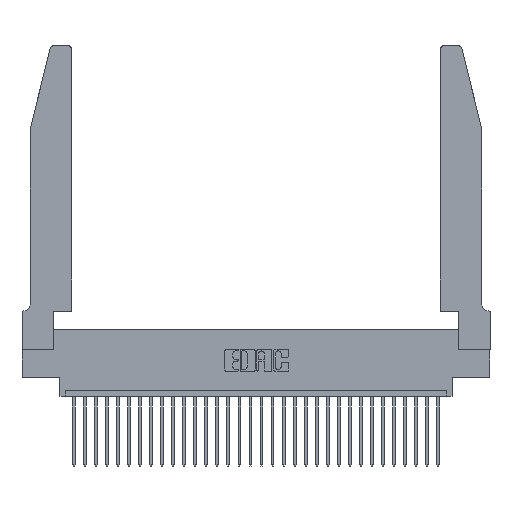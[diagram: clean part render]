
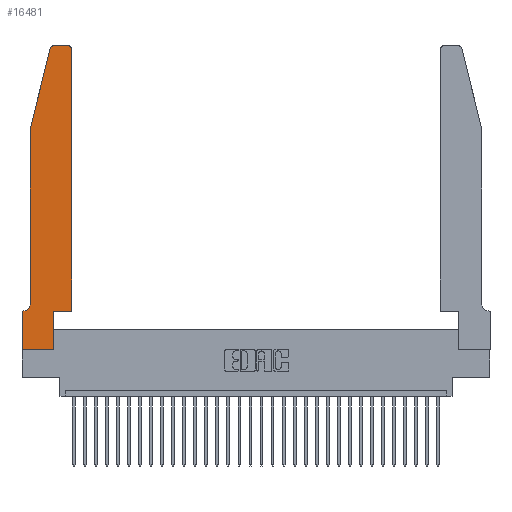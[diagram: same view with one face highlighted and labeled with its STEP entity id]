
A CAD part, top view. The second image highlights one B-rep face of the part: STEP entity #16481.
In plain terms, the highlighted planar face has unit normal (0, 0, 1).
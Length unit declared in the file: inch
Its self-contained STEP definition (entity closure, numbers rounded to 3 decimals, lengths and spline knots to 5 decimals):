
#153 = CARTESIAN_POINT ( 'NONE',  ( 0.0755, 2., 0.37 ) ) ;
#280 = CARTESIAN_POINT ( 'NONE',  ( 0.0055, 0.35, 0.37 ) ) ;
#461 = CIRCLE ( 'NONE', #27323, 0.07 ) ;
#465 = EDGE_CURVE ( 'NONE', #18346, #7004, #461, .T. ) ;
#508 = CARTESIAN_POINT ( 'NONE',  ( 0.284, 2.75, 0.37 ) ) ;
#519 = CARTESIAN_POINT ( 'NONE',  ( 0.2865, 0.35, 0.37 ) ) ;
#1228 = CARTESIAN_POINT ( 'NONE',  ( 0., 0., 0.37 ) ) ;
#1520 = VERTEX_POINT ( 'NONE', #13369 ) ;
#1771 = VECTOR ( 'NONE', #6587, 39.37008 ) ;
#2228 = CARTESIAN_POINT ( 'NONE',  ( 0.2865, 0., 0.37 ) ) ;
#2359 = DIRECTION ( 'NONE',  ( 0., 1., 0. ) ) ;
#2388 = EDGE_CURVE ( 'NONE', #21595, #28389, #28899, .T. ) ;
#2615 = CARTESIAN_POINT ( 'NONE',  ( 0.4205, 2.75, 0.37 ) ) ;
#2715 = DIRECTION ( 'NONE',  ( 1., 0., 0. ) ) ;
#3017 = DIRECTION ( 'NONE',  ( 0., 0., 1. ) ) ;
#3355 = CARTESIAN_POINT ( 'NONE',  ( 0., 0., 0.37 ) ) ;
#3559 = FACE_OUTER_BOUND ( 'NONE', #24918, .T. ) ;
#3986 = ORIENTED_EDGE ( 'NONE', *, *, #2388, .T. ) ;
#4025 = EDGE_CURVE ( 'NONE', #29875, #5125, #22095, .T. ) ;
#4460 = CARTESIAN_POINT ( 'NONE',  ( 0., 0.35, 0.37 ) ) ;
#4710 = AXIS2_PLACEMENT_3D ( 'NONE', #29635, #3017, #22829 ) ;
#4924 = VECTOR ( 'NONE', #28010, 39.37008 ) ;
#5125 = VERTEX_POINT ( 'NONE', #508 ) ;
#5462 = DIRECTION ( 'NONE',  ( 1., 0., 0. ) ) ;
#5495 = CIRCLE ( 'NONE', #13452, 0.03 ) ;
#5719 = CARTESIAN_POINT ( 'NONE',  ( 0.0755, 2., 0.37 ) ) ;
#5779 = DIRECTION ( 'NONE',  ( 0., -1., 0. ) ) ;
#6279 = EDGE_CURVE ( 'NONE', #29318, #1520, #27963, .T. ) ;
#6471 = CARTESIAN_POINT ( 'NONE',  ( 0.25487, 2.72718, 0.37 ) ) ;
#6587 = DIRECTION ( 'NONE',  ( -0.239, -0.971, 0. ) ) ;
#7004 = VERTEX_POINT ( 'NONE', #280 ) ;
#7133 = CARTESIAN_POINT ( 'NONE',  ( 0.4505, 0.35, 0.37 ) ) ;
#7523 = CARTESIAN_POINT ( 'NONE',  ( 0.284, 2.72, 0.37 ) ) ;
#8044 = CARTESIAN_POINT ( 'NONE',  ( 0.0755, 2., 0.37 ) ) ;
#8308 = CARTESIAN_POINT ( 'NONE',  ( 0.2865, 0.35, 0.37 ) ) ;
#8574 = VECTOR ( 'NONE', #5462, 39.37008 ) ;
#8575 = DIRECTION ( 'NONE',  ( 1., 0., 0. ) ) ;
#10218 = ORIENTED_EDGE ( 'NONE', *, *, #6279, .T. ) ;
#10590 = EDGE_CURVE ( 'NONE', #17412, #28725, #29959, .T. ) ;
#11073 = CARTESIAN_POINT ( 'NONE',  ( 0.2605, 2.75, 0.37 ) ) ;
#11079 = DIRECTION ( 'NONE',  ( -1., 0., 0. ) ) ;
#11235 = ORIENTED_EDGE ( 'NONE', *, *, #23697, .T. ) ;
#11522 = VERTEX_POINT ( 'NONE', #23564 ) ;
#11557 = LINE ( 'NONE', #3355, #29860 ) ;
#12102 = EDGE_CURVE ( 'NONE', #1520, #29875, #18906, .T. ) ;
#12109 = EDGE_CURVE ( 'NONE', #13665, #29318, #15053, .T. ) ;
#12166 = CARTESIAN_POINT ( 'NONE',  ( 0., 0., 0.37 ) ) ;
#12232 = AXIS2_PLACEMENT_3D ( 'NONE', #4460, #28842, #24043 ) ;
#12554 = VECTOR ( 'NONE', #14605, 39.37008 ) ;
#12715 = CARTESIAN_POINT ( 'NONE',  ( 0.0755, 0.42, 0.37 ) ) ;
#12849 = CARTESIAN_POINT ( 'NONE',  ( 0.4505, 0.35, 0.37 ) ) ;
#13369 = CARTESIAN_POINT ( 'NONE',  ( 0.4505, 2.72, 0.37 ) ) ;
#13452 = AXIS2_PLACEMENT_3D ( 'NONE', #7523, #22052, #2715 ) ;
#13665 = VERTEX_POINT ( 'NONE', #519 ) ;
#14605 = DIRECTION ( 'NONE',  ( 0., -1., 0. ) ) ;
#14784 = VECTOR ( 'NONE', #28127, 39.37008 ) ;
#15053 = LINE ( 'NONE', #12849, #8574 ) ;
#15321 = ORIENTED_EDGE ( 'NONE', *, *, #10590, .T. ) ;
#15621 = ORIENTED_EDGE ( 'NONE', *, *, #12109, .T. ) ;
#15746 = CARTESIAN_POINT ( 'NONE',  ( 0.0755, 0.35, 0.37 ) ) ;
#15978 = DIRECTION ( 'NONE',  ( 0., 0., -1. ) ) ;
#16303 = VECTOR ( 'NONE', #8575, 39.37008 ) ;
#16481 = ADVANCED_FACE ( 'NONE', ( #3559 ), #28945, .T. ) ;
#17412 = VERTEX_POINT ( 'NONE', #6471 ) ;
#18205 = VECTOR ( 'NONE', #20662, 39.37008 ) ;
#18346 = VERTEX_POINT ( 'NONE', #12715 ) ;
#18906 = CIRCLE ( 'NONE', #4710, 0.03 ) ;
#19508 = CARTESIAN_POINT ( 'NONE',  ( 0.4505, 0.35, 0.37 ) ) ;
#20043 = ORIENTED_EDGE ( 'NONE', *, *, #29985, .T. ) ;
#20564 = ORIENTED_EDGE ( 'NONE', *, *, #23093, .T. ) ;
#20662 = DIRECTION ( 'NONE',  ( -1., 0., 0. ) ) ;
#21595 = VERTEX_POINT ( 'NONE', #12166 ) ;
#22018 = EDGE_CURVE ( 'NONE', #28725, #18346, #25561, .T. ) ;
#22052 = DIRECTION ( 'NONE',  ( 0., 0., 1. ) ) ;
#22095 = LINE ( 'NONE', #11073, #14784 ) ;
#22303 = ORIENTED_EDGE ( 'NONE', *, *, #4025, .T. ) ;
#22824 = LINE ( 'NONE', #8308, #4924 ) ;
#22829 = DIRECTION ( 'NONE',  ( 1., 0., 0. ) ) ;
#23093 = EDGE_CURVE ( 'NONE', #28389, #13665, #22824, .T. ) ;
#23564 = CARTESIAN_POINT ( 'NONE',  ( 0., 0.35, 0.37 ) ) ;
#23697 = EDGE_CURVE ( 'NONE', #7004, #11522, #25433, .T. ) ;
#24043 = DIRECTION ( 'NONE',  ( 1., 0., 0. ) ) ;
#24099 = ORIENTED_EDGE ( 'NONE', *, *, #465, .T. ) ;
#24918 = EDGE_LOOP ( 'NONE', ( #22303, #26926, #15321, #26862, #24099, #11235, #20043, #3986, #20564, #15621, #10218, #26102 ) ) ;
#25433 = LINE ( 'NONE', #15746, #18205 ) ;
#25561 = LINE ( 'NONE', #153, #12554 ) ;
#26102 = ORIENTED_EDGE ( 'NONE', *, *, #12102, .T. ) ;
#26457 = VECTOR ( 'NONE', #2359, 39.37008 ) ;
#26862 = ORIENTED_EDGE ( 'NONE', *, *, #22018, .T. ) ;
#26926 = ORIENTED_EDGE ( 'NONE', *, *, #29841, .T. ) ;
#27323 = AXIS2_PLACEMENT_3D ( 'NONE', #30574, #15978, #11079 ) ;
#27963 = LINE ( 'NONE', #19508, #26457 ) ;
#28010 = DIRECTION ( 'NONE',  ( 0., 1., 0. ) ) ;
#28127 = DIRECTION ( 'NONE',  ( -1., 0., 0. ) ) ;
#28389 = VERTEX_POINT ( 'NONE', #2228 ) ;
#28725 = VERTEX_POINT ( 'NONE', #8044 ) ;
#28842 = DIRECTION ( 'NONE',  ( 0., 0., 1. ) ) ;
#28899 = LINE ( 'NONE', #1228, #16303 ) ;
#28945 = PLANE ( 'NONE',  #12232 ) ;
#29318 = VERTEX_POINT ( 'NONE', #7133 ) ;
#29635 = CARTESIAN_POINT ( 'NONE',  ( 0.4205, 2.72, 0.37 ) ) ;
#29841 = EDGE_CURVE ( 'NONE', #5125, #17412, #5495, .T. ) ;
#29860 = VECTOR ( 'NONE', #5779, 39.37008 ) ;
#29875 = VERTEX_POINT ( 'NONE', #2615 ) ;
#29959 = LINE ( 'NONE', #5719, #1771 ) ;
#29985 = EDGE_CURVE ( 'NONE', #11522, #21595, #11557, .T. ) ;
#30574 = CARTESIAN_POINT ( 'NONE',  ( 0.0055, 0.42, 0.37 ) ) ;
